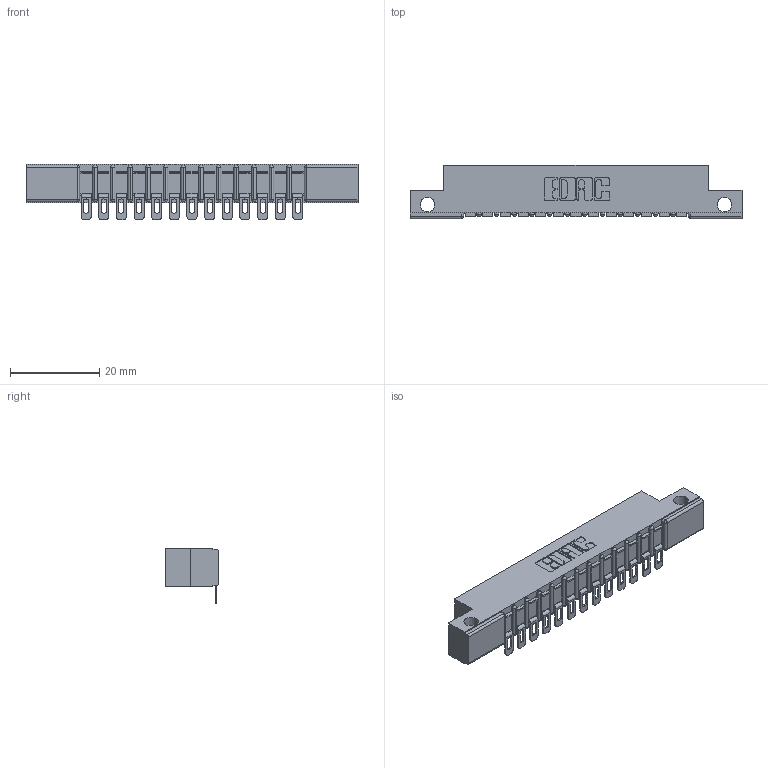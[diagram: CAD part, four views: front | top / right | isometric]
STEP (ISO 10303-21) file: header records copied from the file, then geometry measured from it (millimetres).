
FILE_DESCRIPTION (( 'STEP AP203' ), '1' );
FILE_NAME ('357-013-554-112.STEP', '2018-08-07T23:10:58', ( '' ), ( '' ), 'SwSTEP 2.0', 'SolidWorks 2016', '' );
FILE_SCHEMA (( 'CONFIG_CONTROL_DESIGN' ));
Length unit declared in the file: inch
Products named in the file (3): 307 Part_.128 Dia Side Mounting Holes; 307-290-002_554; 357-013-554-112
Assembly tree (14 placements, depth 2):
  357-013-554-112
    307 Part_.128 Dia Side Mounting Holes
    307-290-002_554  x13
Bounding box: 74.52 x 12.01 x 12.52 mm (x, y, z)
Volume: 4844 mm3; surface area: 8225.9 mm2
Topology: 14 solids, 14 shells, 1185 faces, 3612 edges, 2368 vertices
Faces by surface type: plane 668, cylinder 489, sphere 28
Entity records: 15687 total; most frequent: CARTESIAN_POINT 2642, ORIENTED_EDGE 2632, DIRECTION 2586, EDGE_CURVE 1316, VECTOR 986, LINE 986, VERTEX_POINT 856, AXIS2_PLACEMENT_3D 800
